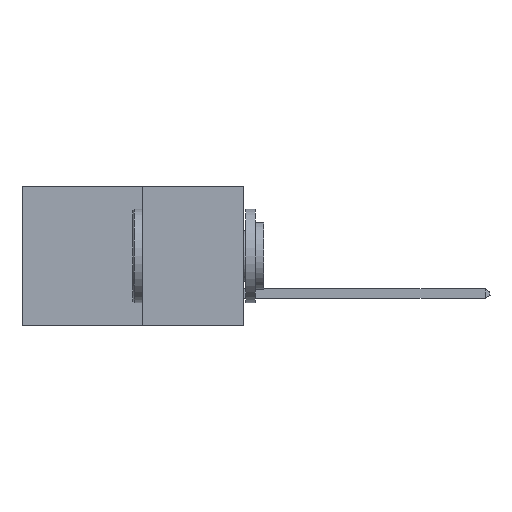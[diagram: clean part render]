
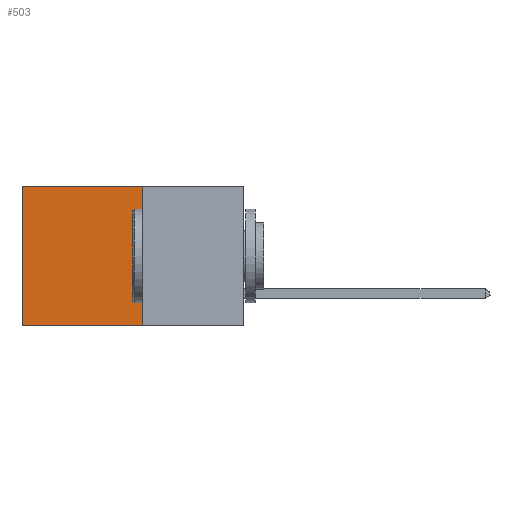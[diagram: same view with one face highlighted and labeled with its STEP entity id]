
A CAD part, left-side view. The second image highlights one B-rep face of the part: STEP entity #503.
In plain terms, the highlighted planar face has unit normal (-1, 0, 0).
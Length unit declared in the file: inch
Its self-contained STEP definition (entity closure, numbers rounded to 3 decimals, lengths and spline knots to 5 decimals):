
#180 = CARTESIAN_POINT ( 'NONE',  ( 0.277, 0.27, -0.37 ) ) ;
#503 = ADVANCED_FACE ( 'NONE', ( #10355 ), #4828, .F. ) ;
#1454 = DIRECTION ( 'NONE',  ( 0., 0., -1. ) ) ;
#2037 = VECTOR ( 'NONE', #4168, 39.37008 ) ;
#3345 = EDGE_LOOP ( 'NONE', ( #14501, #13794, #7852, #9583 ) ) ;
#3808 = DIRECTION ( 'NONE',  ( 0., 0., -1. ) ) ;
#3980 = VECTOR ( 'NONE', #15368, 39.37008 ) ;
#4116 = CARTESIAN_POINT ( 'NONE',  ( 0.277, 0.27, 0. ) ) ;
#4168 = DIRECTION ( 'NONE',  ( 0., 1., 0. ) ) ;
#4472 = CARTESIAN_POINT ( 'NONE',  ( 0.277, 0.27, -0.37 ) ) ;
#4768 = CARTESIAN_POINT ( 'NONE',  ( 0.277, 0.59, 0. ) ) ;
#4828 = PLANE ( 'NONE',  #14543 ) ;
#4908 = DIRECTION ( 'NONE',  ( 0., 0., -1. ) ) ;
#5366 = LINE ( 'NONE', #4116, #2037 ) ;
#6596 = DIRECTION ( 'NONE',  ( 1., 0., 0. ) ) ;
#6658 = VERTEX_POINT ( 'NONE', #6863 ) ;
#6753 = CARTESIAN_POINT ( 'NONE',  ( 0.277, 0.27, -0.37 ) ) ;
#6863 = CARTESIAN_POINT ( 'NONE',  ( 0.277, 0.27, 0. ) ) ;
#7624 = EDGE_CURVE ( 'NONE', #6658, #8687, #5366, .T. ) ;
#7852 = ORIENTED_EDGE ( 'NONE', *, *, #11533, .F. ) ;
#8191 = VERTEX_POINT ( 'NONE', #13786 ) ;
#8411 = EDGE_CURVE ( 'NONE', #9159, #8191, #10983, .T. ) ;
#8687 = VERTEX_POINT ( 'NONE', #4768 ) ;
#9159 = VERTEX_POINT ( 'NONE', #10916 ) ;
#9324 = VECTOR ( 'NONE', #1454, 39.37008 ) ;
#9583 = ORIENTED_EDGE ( 'NONE', *, *, #7624, .T. ) ;
#9866 = CARTESIAN_POINT ( 'NONE',  ( 0.277, 0.59, -0.37 ) ) ;
#10355 = FACE_OUTER_BOUND ( 'NONE', #3345, .T. ) ;
#10916 = CARTESIAN_POINT ( 'NONE',  ( 0.277, 0.27, -0.37 ) ) ;
#10983 = LINE ( 'NONE', #6753, #3980 ) ;
#11347 = EDGE_CURVE ( 'NONE', #8687, #8191, #11661, .T. ) ;
#11533 = EDGE_CURVE ( 'NONE', #6658, #9159, #15841, .T. ) ;
#11661 = LINE ( 'NONE', #9866, #14521 ) ;
#13786 = CARTESIAN_POINT ( 'NONE',  ( 0.277, 0.59, -0.37 ) ) ;
#13794 = ORIENTED_EDGE ( 'NONE', *, *, #8411, .F. ) ;
#14501 = ORIENTED_EDGE ( 'NONE', *, *, #11347, .T. ) ;
#14521 = VECTOR ( 'NONE', #4908, 39.37008 ) ;
#14543 = AXIS2_PLACEMENT_3D ( 'NONE', #4472, #6596, #3808 ) ;
#15368 = DIRECTION ( 'NONE',  ( 0., 1., 0. ) ) ;
#15841 = LINE ( 'NONE', #180, #9324 ) ;
